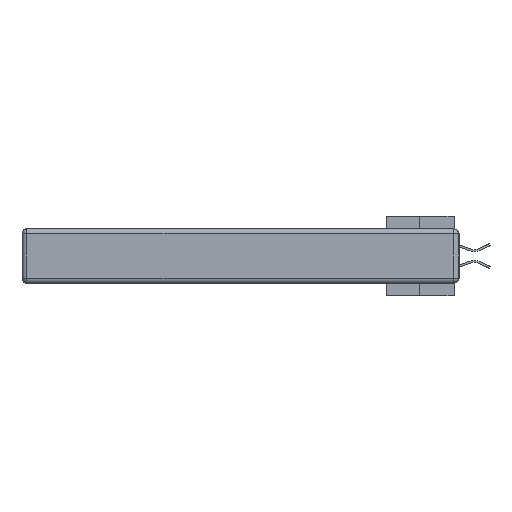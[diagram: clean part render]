
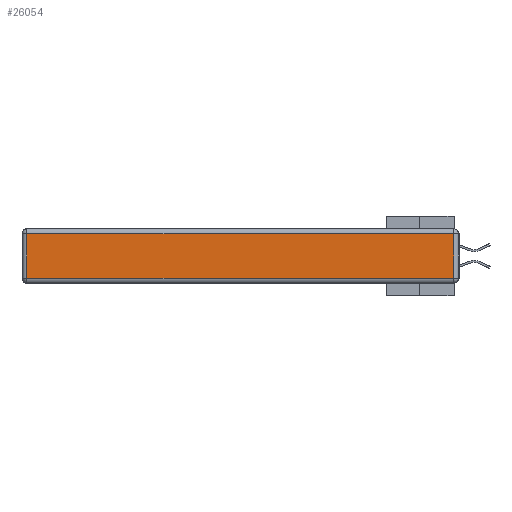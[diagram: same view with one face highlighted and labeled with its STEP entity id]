
A CAD part, left-side view. The second image highlights one B-rep face of the part: STEP entity #26054.
In plain terms, the highlighted planar face has unit normal (-1, 0, 0).
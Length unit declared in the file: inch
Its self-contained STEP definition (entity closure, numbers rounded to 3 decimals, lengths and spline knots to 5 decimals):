
#1103 = LINE ( 'NONE', #9243, #3124 ) ;
#1764 = EDGE_CURVE ( 'NONE', #26820, #26862, #21919, .T. ) ;
#3124 = VECTOR ( 'NONE', #12151, 39.37008 ) ;
#3140 = FACE_OUTER_BOUND ( 'NONE', #31516, .T. ) ;
#4123 = CARTESIAN_POINT ( 'NONE',  ( 0., 0.03, -0.03 ) ) ;
#4775 = CARTESIAN_POINT ( 'NONE',  ( 0., 2.72, -0.03 ) ) ;
#6664 = CARTESIAN_POINT ( 'NONE',  ( 0., 0., -0.343 ) ) ;
#6957 = DIRECTION ( 'NONE',  ( -1., 0., 0. ) ) ;
#7213 = DIRECTION ( 'NONE',  ( 0., 1., 0. ) ) ;
#7265 = DIRECTION ( 'NONE',  ( 0., -1., 0. ) ) ;
#7774 = CARTESIAN_POINT ( 'NONE',  ( 0., 0.03, -0.343 ) ) ;
#8304 = VERTEX_POINT ( 'NONE', #4123 ) ;
#9243 = CARTESIAN_POINT ( 'NONE',  ( 0., 2.72, -0.343 ) ) ;
#10721 = LINE ( 'NONE', #15839, #26691 ) ;
#12151 = DIRECTION ( 'NONE',  ( 0., 0., -1. ) ) ;
#12502 = ORIENTED_EDGE ( 'NONE', *, *, #22995, .T. ) ;
#12512 = CARTESIAN_POINT ( 'NONE',  ( 0., 0.03, -0.313 ) ) ;
#15634 = LINE ( 'NONE', #7774, #23383 ) ;
#15839 = CARTESIAN_POINT ( 'NONE',  ( 0., 2.75, -0.03 ) ) ;
#20131 = EDGE_CURVE ( 'NONE', #36562, #26820, #1103, .T. ) ;
#20998 = DIRECTION ( 'NONE',  ( 0., 0., 1. ) ) ;
#21919 = LINE ( 'NONE', #39951, #26019 ) ;
#22995 = EDGE_CURVE ( 'NONE', #8304, #36562, #10721, .T. ) ;
#23276 = AXIS2_PLACEMENT_3D ( 'NONE', #6664, #6957, #26379 ) ;
#23383 = VECTOR ( 'NONE', #20998, 39.37008 ) ;
#26019 = VECTOR ( 'NONE', #7265, 39.37008 ) ;
#26054 = ADVANCED_FACE ( 'NONE', ( #3140 ), #26689, .T. ) ;
#26379 = DIRECTION ( 'NONE',  ( 0., 0., 1. ) ) ;
#26689 = PLANE ( 'NONE',  #23276 ) ;
#26691 = VECTOR ( 'NONE', #7213, 39.37008 ) ;
#26820 = VERTEX_POINT ( 'NONE', #34778 ) ;
#26862 = VERTEX_POINT ( 'NONE', #12512 ) ;
#28997 = ORIENTED_EDGE ( 'NONE', *, *, #31976, .T. ) ;
#31516 = EDGE_LOOP ( 'NONE', ( #32381, #28997, #12502, #34945 ) ) ;
#31976 = EDGE_CURVE ( 'NONE', #26862, #8304, #15634, .T. ) ;
#32381 = ORIENTED_EDGE ( 'NONE', *, *, #1764, .T. ) ;
#34778 = CARTESIAN_POINT ( 'NONE',  ( 0., 2.72, -0.313 ) ) ;
#34945 = ORIENTED_EDGE ( 'NONE', *, *, #20131, .T. ) ;
#36562 = VERTEX_POINT ( 'NONE', #4775 ) ;
#39951 = CARTESIAN_POINT ( 'NONE',  ( 0., 0., -0.313 ) ) ;
